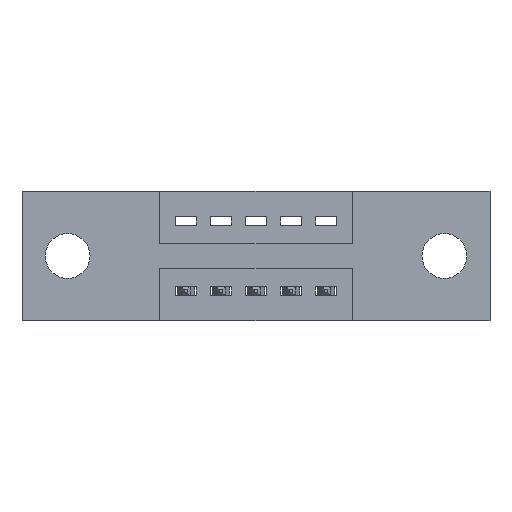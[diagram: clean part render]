
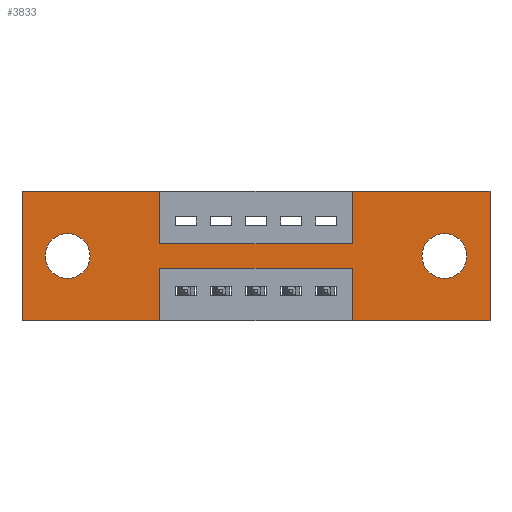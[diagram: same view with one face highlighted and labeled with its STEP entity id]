
A CAD part, front view. The second image highlights one B-rep face of the part: STEP entity #3833.
In plain terms, the highlighted planar face has unit normal (0, -1, 0).
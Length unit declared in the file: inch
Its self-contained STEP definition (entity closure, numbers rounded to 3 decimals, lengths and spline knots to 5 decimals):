
#42 = VERTEX_POINT ( 'NONE', #3481 ) ;
#67 = FACE_BOUND ( 'NONE', #7101, .T. ) ;
#184 = EDGE_CURVE ( 'NONE', #7032, #2815, #3744, .T. ) ;
#252 = CARTESIAN_POINT ( 'NONE',  ( 0., 0., -0.37 ) ) ;
#418 = AXIS2_PLACEMENT_3D ( 'NONE', #1971, #2688, #4801 ) ;
#485 = PLANE ( 'NONE',  #418 ) ;
#518 = ORIENTED_EDGE ( 'NONE', *, *, #3382, .F. ) ;
#608 = DIRECTION ( 'NONE',  ( 0., 1., 0. ) ) ;
#688 = EDGE_CURVE ( 'NONE', #3774, #7032, #7195, .T. ) ;
#753 = CARTESIAN_POINT ( 'NONE',  ( 1.205, 0., -0.121 ) ) ;
#1005 = VERTEX_POINT ( 'NONE', #8219 ) ;
#1017 = EDGE_LOOP ( 'NONE', ( #7855, #4351, #4384, #7070, #4509, #2014, #4672, #4590, #518, #3728, #4691, #7336 ) ) ;
#1042 = EDGE_CURVE ( 'NONE', #6615, #6320, #1806, .T. ) ;
#1059 = CARTESIAN_POINT ( 'NONE',  ( 0., 0., 0. ) ) ;
#1074 = DIRECTION ( 'NONE',  ( 1., 0., 0. ) ) ;
#1075 = LINE ( 'NONE', #1230, #3823 ) ;
#1084 = CARTESIAN_POINT ( 'NONE',  ( 0.3925, 0., -0.22 ) ) ;
#1148 = LINE ( 'NONE', #8147, #1363 ) ;
#1197 = DIRECTION ( 'NONE',  ( 0., 0., -1. ) ) ;
#1230 = CARTESIAN_POINT ( 'NONE',  ( 0.3925, 0., -0.37 ) ) ;
#1252 = EDGE_CURVE ( 'NONE', #8477, #6615, #1075, .T. ) ;
#1318 = CARTESIAN_POINT ( 'NONE',  ( 0., 0., 0. ) ) ;
#1363 = VECTOR ( 'NONE', #7550, 39.37008 ) ;
#1365 = EDGE_CURVE ( 'NONE', #4034, #4568, #2659, .T. ) ;
#1507 = EDGE_CURVE ( 'NONE', #3436, #3020, #3411, .T. ) ;
#1560 = DIRECTION ( 'NONE',  ( -1., 0., 0. ) ) ;
#1639 = CARTESIAN_POINT ( 'NONE',  ( 0.9425, 0., -0.37 ) ) ;
#1689 = CARTESIAN_POINT ( 'NONE',  ( 0.13, 0., -0.249 ) ) ;
#1806 = LINE ( 'NONE', #252, #6769 ) ;
#1881 = CARTESIAN_POINT ( 'NONE',  ( 0.3925, 0., -0.15 ) ) ;
#1921 = VECTOR ( 'NONE', #1074, 39.37008 ) ;
#1971 = CARTESIAN_POINT ( 'NONE',  ( 0., 0., -0.37 ) ) ;
#2014 = ORIENTED_EDGE ( 'NONE', *, *, #5923, .F. ) ;
#2066 = CARTESIAN_POINT ( 'NONE',  ( 0.9425, 0., 0. ) ) ;
#2165 = CARTESIAN_POINT ( 'NONE',  ( 1.335, 0., -0.37 ) ) ;
#2286 = CARTESIAN_POINT ( 'NONE',  ( 1.205, 0., -0.249 ) ) ;
#2323 = CARTESIAN_POINT ( 'NONE',  ( 0.9425, 0., 0. ) ) ;
#2659 = LINE ( 'NONE', #7287, #3189 ) ;
#2688 = DIRECTION ( 'NONE',  ( 0., -1., 0. ) ) ;
#2714 = ORIENTED_EDGE ( 'NONE', *, *, #4676, .T. ) ;
#2748 = AXIS2_PLACEMENT_3D ( 'NONE', #6982, #7664, #3639 ) ;
#2815 = VERTEX_POINT ( 'NONE', #2066 ) ;
#2919 = VECTOR ( 'NONE', #6019, 39.37008 ) ;
#2962 = EDGE_CURVE ( 'NONE', #4568, #1005, #1148, .T. ) ;
#3020 = VERTEX_POINT ( 'NONE', #2286 ) ;
#3033 = CIRCLE ( 'NONE', #3564, 0.064 ) ;
#3189 = VECTOR ( 'NONE', #3274, 39.37008 ) ;
#3221 = CARTESIAN_POINT ( 'NONE',  ( 0.3925, 0., -0.15 ) ) ;
#3234 = CARTESIAN_POINT ( 'NONE',  ( 0.3925, 0., 0. ) ) ;
#3274 = DIRECTION ( 'NONE',  ( -1., 0., 0. ) ) ;
#3342 = LINE ( 'NONE', #1318, #2919 ) ;
#3382 = EDGE_CURVE ( 'NONE', #4816, #3774, #4413, .T. ) ;
#3411 = CIRCLE ( 'NONE', #6791, 0.064 ) ;
#3436 = VERTEX_POINT ( 'NONE', #753 ) ;
#3475 = FACE_OUTER_BOUND ( 'NONE', #1017, .T. ) ;
#3481 = CARTESIAN_POINT ( 'NONE',  ( 1.335, 0., 0. ) ) ;
#3564 = AXIS2_PLACEMENT_3D ( 'NONE', #3770, #4428, #7164 ) ;
#3639 = DIRECTION ( 'NONE',  ( 0., 0., 1. ) ) ;
#3728 = ORIENTED_EDGE ( 'NONE', *, *, #4749, .F. ) ;
#3735 = EDGE_CURVE ( 'NONE', #7041, #7252, #6203, .T. ) ;
#3744 = LINE ( 'NONE', #2323, #5305 ) ;
#3770 = CARTESIAN_POINT ( 'NONE',  ( 1.205, 0., -0.185 ) ) ;
#3774 = VERTEX_POINT ( 'NONE', #1881 ) ;
#3788 = DIRECTION ( 'NONE',  ( 1., 0., 0. ) ) ;
#3823 = VECTOR ( 'NONE', #5840, 39.37008 ) ;
#3833 = ADVANCED_FACE ( 'NONE', ( #67, #6608, #3475 ), #485, .T. ) ;
#3838 = ORIENTED_EDGE ( 'NONE', *, *, #8269, .T. ) ;
#3931 = DIRECTION ( 'NONE',  ( 0., 0., -1. ) ) ;
#4034 = VERTEX_POINT ( 'NONE', #2165 ) ;
#4091 = VECTOR ( 'NONE', #1560, 39.37008 ) ;
#4302 = DIRECTION ( 'NONE',  ( 0., 1., 0. ) ) ;
#4351 = ORIENTED_EDGE ( 'NONE', *, *, #6275, .F. ) ;
#4384 = ORIENTED_EDGE ( 'NONE', *, *, #2962, .F. ) ;
#4413 = LINE ( 'NONE', #7261, #8754 ) ;
#4428 = DIRECTION ( 'NONE',  ( 0., 1., 0. ) ) ;
#4509 = ORIENTED_EDGE ( 'NONE', *, *, #8023, .F. ) ;
#4550 = VECTOR ( 'NONE', #3788, 39.37008 ) ;
#4568 = VERTEX_POINT ( 'NONE', #1639 ) ;
#4590 = ORIENTED_EDGE ( 'NONE', *, *, #688, .F. ) ;
#4672 = ORIENTED_EDGE ( 'NONE', *, *, #184, .F. ) ;
#4676 = EDGE_CURVE ( 'NONE', #3020, #3436, #3033, .T. ) ;
#4691 = ORIENTED_EDGE ( 'NONE', *, *, #7183, .F. ) ;
#4749 = EDGE_CURVE ( 'NONE', #7204, #4816, #4779, .T. ) ;
#4779 = LINE ( 'NONE', #5168, #1921 ) ;
#4789 = CARTESIAN_POINT ( 'NONE',  ( 0.13, 0., -0.121 ) ) ;
#4801 = DIRECTION ( 'NONE',  ( 0., 0., -1. ) ) ;
#4816 = VERTEX_POINT ( 'NONE', #3234 ) ;
#4966 = CARTESIAN_POINT ( 'NONE',  ( 0.3925, 0., -0.22 ) ) ;
#5127 = ORIENTED_EDGE ( 'NONE', *, *, #3735, .T. ) ;
#5168 = CARTESIAN_POINT ( 'NONE',  ( 0., 0., 0. ) ) ;
#5305 = VECTOR ( 'NONE', #7701, 39.37008 ) ;
#5811 = DIRECTION ( 'NONE',  ( 1., 0., 0. ) ) ;
#5840 = DIRECTION ( 'NONE',  ( 0., 0., -1. ) ) ;
#5923 = EDGE_CURVE ( 'NONE', #2815, #42, #7672, .T. ) ;
#6019 = DIRECTION ( 'NONE',  ( 0., 0., 1. ) ) ;
#6203 = CIRCLE ( 'NONE', #7250, 0.064 ) ;
#6275 = EDGE_CURVE ( 'NONE', #1005, #8477, #7771, .T. ) ;
#6320 = VERTEX_POINT ( 'NONE', #6883 ) ;
#6370 = DIRECTION ( 'NONE',  ( -1., 0., 0. ) ) ;
#6450 = DIRECTION ( 'NONE',  ( 0., 0., -1. ) ) ;
#6543 = DIRECTION ( 'NONE',  ( 0., 0., 1. ) ) ;
#6608 = FACE_BOUND ( 'NONE', #7377, .T. ) ;
#6610 = VECTOR ( 'NONE', #5811, 39.37008 ) ;
#6615 = VERTEX_POINT ( 'NONE', #7375 ) ;
#6769 = VECTOR ( 'NONE', #6370, 39.37008 ) ;
#6791 = AXIS2_PLACEMENT_3D ( 'NONE', #8294, #4302, #6450 ) ;
#6883 = CARTESIAN_POINT ( 'NONE',  ( 0., 0., -0.37 ) ) ;
#6899 = ORIENTED_EDGE ( 'NONE', *, *, #1507, .T. ) ;
#6982 = CARTESIAN_POINT ( 'NONE',  ( 0.13, 0., -0.185 ) ) ;
#7032 = VERTEX_POINT ( 'NONE', #7125 ) ;
#7041 = VERTEX_POINT ( 'NONE', #1689 ) ;
#7070 = ORIENTED_EDGE ( 'NONE', *, *, #1365, .F. ) ;
#7089 = CIRCLE ( 'NONE', #2748, 0.064 ) ;
#7101 = EDGE_LOOP ( 'NONE', ( #6899, #2714 ) ) ;
#7125 = CARTESIAN_POINT ( 'NONE',  ( 0.9425, 0., -0.15 ) ) ;
#7164 = DIRECTION ( 'NONE',  ( 0., 0., -1. ) ) ;
#7183 = EDGE_CURVE ( 'NONE', #6320, #7204, #3342, .T. ) ;
#7195 = LINE ( 'NONE', #3221, #4550 ) ;
#7204 = VERTEX_POINT ( 'NONE', #7441 ) ;
#7250 = AXIS2_PLACEMENT_3D ( 'NONE', #8625, #608, #6543 ) ;
#7252 = VERTEX_POINT ( 'NONE', #4789 ) ;
#7261 = CARTESIAN_POINT ( 'NONE',  ( 0.3925, 0., 0. ) ) ;
#7287 = CARTESIAN_POINT ( 'NONE',  ( 0., 0., -0.37 ) ) ;
#7309 = VECTOR ( 'NONE', #3931, 39.37008 ) ;
#7336 = ORIENTED_EDGE ( 'NONE', *, *, #1042, .F. ) ;
#7375 = CARTESIAN_POINT ( 'NONE',  ( 0.3925, 0., -0.37 ) ) ;
#7377 = EDGE_LOOP ( 'NONE', ( #3838, #5127 ) ) ;
#7441 = CARTESIAN_POINT ( 'NONE',  ( 0., 0., 0. ) ) ;
#7550 = DIRECTION ( 'NONE',  ( 0., 0., 1. ) ) ;
#7664 = DIRECTION ( 'NONE',  ( 0., 1., 0. ) ) ;
#7672 = LINE ( 'NONE', #1059, #6610 ) ;
#7701 = DIRECTION ( 'NONE',  ( 0., 0., 1. ) ) ;
#7771 = LINE ( 'NONE', #4966, #4091 ) ;
#7855 = ORIENTED_EDGE ( 'NONE', *, *, #1252, .F. ) ;
#7965 = CARTESIAN_POINT ( 'NONE',  ( 1.335, 0., 0. ) ) ;
#8023 = EDGE_CURVE ( 'NONE', #42, #4034, #8499, .T. ) ;
#8147 = CARTESIAN_POINT ( 'NONE',  ( 0.9425, 0., -0.37 ) ) ;
#8219 = CARTESIAN_POINT ( 'NONE',  ( 0.9425, 0., -0.22 ) ) ;
#8269 = EDGE_CURVE ( 'NONE', #7252, #7041, #7089, .T. ) ;
#8294 = CARTESIAN_POINT ( 'NONE',  ( 1.205, 0., -0.185 ) ) ;
#8477 = VERTEX_POINT ( 'NONE', #1084 ) ;
#8499 = LINE ( 'NONE', #7965, #7309 ) ;
#8625 = CARTESIAN_POINT ( 'NONE',  ( 0.13, 0., -0.185 ) ) ;
#8754 = VECTOR ( 'NONE', #1197, 39.37008 ) ;
